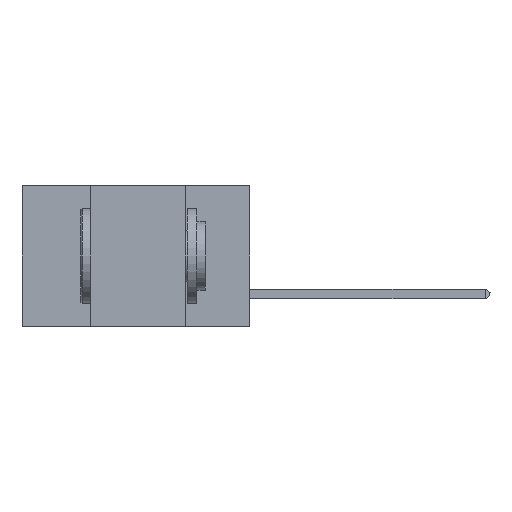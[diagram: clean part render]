
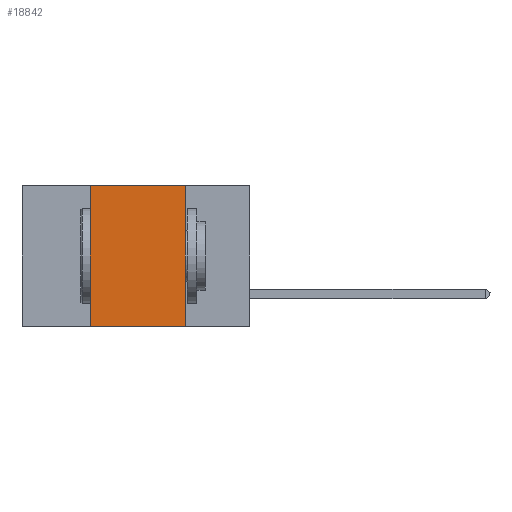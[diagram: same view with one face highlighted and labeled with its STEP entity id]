
A CAD part, left-side view. The second image highlights one B-rep face of the part: STEP entity #18842.
In plain terms, the highlighted planar face has unit normal (-1, 0, 0).
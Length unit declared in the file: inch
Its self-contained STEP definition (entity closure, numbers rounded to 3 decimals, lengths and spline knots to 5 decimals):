
#1451 = DIRECTION ( 'NONE',  ( 0., 0., -1. ) ) ;
#1840 = CARTESIAN_POINT ( 'NONE',  ( 0., 0.17, -0.37 ) ) ;
#1850 = DIRECTION ( 'NONE',  ( 0., 0., -1. ) ) ;
#2133 = CARTESIAN_POINT ( 'NONE',  ( 0., 0.17, 0. ) ) ;
#2707 = ORIENTED_EDGE ( 'NONE', *, *, #6886, .F. ) ;
#4867 = ORIENTED_EDGE ( 'NONE', *, *, #10566, .T. ) ;
#4982 = PLANE ( 'NONE',  #35593 ) ;
#5849 = CARTESIAN_POINT ( 'NONE',  ( 0., 0.42, -0.37 ) ) ;
#6858 = VERTEX_POINT ( 'NONE', #2133 ) ;
#6886 = EDGE_CURVE ( 'NONE', #6858, #7582, #10521, .T. ) ;
#7582 = VERTEX_POINT ( 'NONE', #1840 ) ;
#9836 = VECTOR ( 'NONE', #26726, 39.37008 ) ;
#10521 = LINE ( 'NONE', #21136, #21112 ) ;
#10566 = EDGE_CURVE ( 'NONE', #30217, #7582, #16341, .T. ) ;
#10952 = VECTOR ( 'NONE', #23335, 39.37008 ) ;
#11505 = LINE ( 'NONE', #31175, #10952 ) ;
#13839 = EDGE_LOOP ( 'NONE', ( #2707, #14366, #31324, #4867 ) ) ;
#14276 = CARTESIAN_POINT ( 'NONE',  ( 0., 0.6, 0. ) ) ;
#14366 = ORIENTED_EDGE ( 'NONE', *, *, #16748, .F. ) ;
#16341 = LINE ( 'NONE', #22927, #9836 ) ;
#16748 = EDGE_CURVE ( 'NONE', #36175, #6858, #11505, .T. ) ;
#17831 = FACE_OUTER_BOUND ( 'NONE', #13839, .T. ) ;
#18842 = ADVANCED_FACE ( 'NONE', ( #17831 ), #4982, .F. ) ;
#20697 = CARTESIAN_POINT ( 'NONE',  ( 0., 0.42, 0. ) ) ;
#20840 = DIRECTION ( 'NONE',  ( 0., 0., 1. ) ) ;
#21112 = VECTOR ( 'NONE', #1850, 39.37008 ) ;
#21118 = LINE ( 'NONE', #20697, #35729 ) ;
#21136 = CARTESIAN_POINT ( 'NONE',  ( 0., 0.17, 0. ) ) ;
#22927 = CARTESIAN_POINT ( 'NONE',  ( 0., 0.6, -0.37 ) ) ;
#23256 = EDGE_CURVE ( 'NONE', #30217, #36175, #21118, .T. ) ;
#23335 = DIRECTION ( 'NONE',  ( 0., -1., 0. ) ) ;
#26726 = DIRECTION ( 'NONE',  ( 0., -1., 0. ) ) ;
#30217 = VERTEX_POINT ( 'NONE', #5849 ) ;
#31175 = CARTESIAN_POINT ( 'NONE',  ( 0., 0.6, 0. ) ) ;
#31324 = ORIENTED_EDGE ( 'NONE', *, *, #23256, .F. ) ;
#33852 = DIRECTION ( 'NONE',  ( 1., 0., 0. ) ) ;
#35593 = AXIS2_PLACEMENT_3D ( 'NONE', #14276, #33852, #1451 ) ;
#35729 = VECTOR ( 'NONE', #20840, 39.37008 ) ;
#36175 = VERTEX_POINT ( 'NONE', #36628 ) ;
#36628 = CARTESIAN_POINT ( 'NONE',  ( 0., 0.42, 0. ) ) ;
